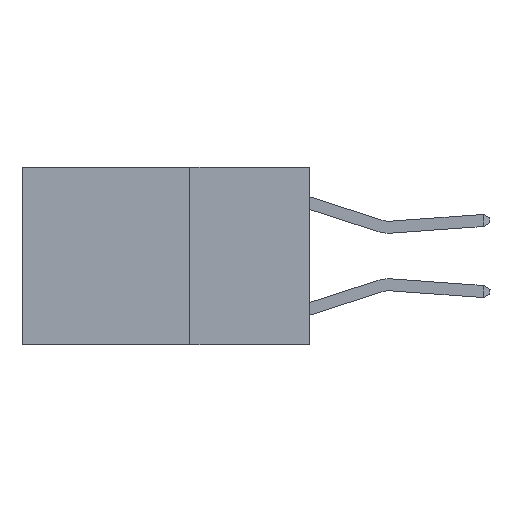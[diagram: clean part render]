
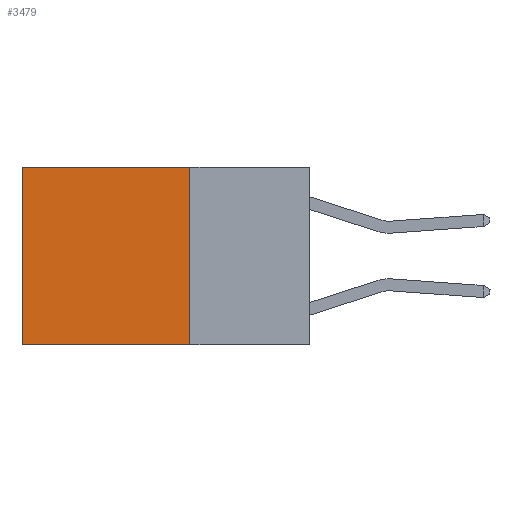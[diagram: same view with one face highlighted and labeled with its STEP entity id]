
A CAD part, left-side view. The second image highlights one B-rep face of the part: STEP entity #3479.
In plain terms, the highlighted planar face has unit normal (-1, 0, 0).
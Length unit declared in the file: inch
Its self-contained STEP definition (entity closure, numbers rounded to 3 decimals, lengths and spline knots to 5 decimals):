
#15 = AXIS2_PLACEMENT_3D ( 'NONE', #1675, #5451, #829 ) ;
#39 = PLANE ( 'NONE',  #15 ) ;
#236 = EDGE_CURVE ( 'NONE', #6786, #7391, #913, .T. ) ;
#303 = VERTEX_POINT ( 'NONE', #6705 ) ;
#782 = EDGE_CURVE ( 'NONE', #6786, #303, #9346, .T. ) ;
#812 = ORIENTED_EDGE ( 'NONE', *, *, #9551, .T. ) ;
#829 = DIRECTION ( 'NONE',  ( 0., 0., -1. ) ) ;
#878 = ORIENTED_EDGE ( 'NONE', *, *, #782, .F. ) ;
#913 = LINE ( 'NONE', #9697, #4128 ) ;
#1272 = CARTESIAN_POINT ( 'NONE',  ( 0.2625, 0.25, -0.37 ) ) ;
#1431 = EDGE_CURVE ( 'NONE', #303, #6467, #4686, .T. ) ;
#1623 = ORIENTED_EDGE ( 'NONE', *, *, #236, .T. ) ;
#1675 = CARTESIAN_POINT ( 'NONE',  ( 0.2625, 0.25, 0. ) ) ;
#2903 = VECTOR ( 'NONE', #3567, 39.37008 ) ;
#3479 = ADVANCED_FACE ( 'NONE', ( #6598 ), #39, .F. ) ;
#3567 = DIRECTION ( 'NONE',  ( 0., 1., 0. ) ) ;
#3615 = CARTESIAN_POINT ( 'NONE',  ( 0.2625, 0.6, -0.37 ) ) ;
#3731 = VECTOR ( 'NONE', #3846, 39.37008 ) ;
#3844 = LINE ( 'NONE', #5351, #3731 ) ;
#3846 = DIRECTION ( 'NONE',  ( 0., 0., -1. ) ) ;
#4128 = VECTOR ( 'NONE', #5115, 39.37008 ) ;
#4686 = LINE ( 'NONE', #1272, #2903 ) ;
#5115 = DIRECTION ( 'NONE',  ( 0., 1., 0. ) ) ;
#5351 = CARTESIAN_POINT ( 'NONE',  ( 0.2625, 0.6, 0. ) ) ;
#5451 = DIRECTION ( 'NONE',  ( 1., 0., 0. ) ) ;
#6374 = CARTESIAN_POINT ( 'NONE',  ( 0.2625, 0.6, 0. ) ) ;
#6388 = VECTOR ( 'NONE', #8823, 39.37008 ) ;
#6467 = VERTEX_POINT ( 'NONE', #3615 ) ;
#6598 = FACE_OUTER_BOUND ( 'NONE', #7121, .T. ) ;
#6705 = CARTESIAN_POINT ( 'NONE',  ( 0.2625, 0.25, -0.37 ) ) ;
#6786 = VERTEX_POINT ( 'NONE', #7008 ) ;
#7008 = CARTESIAN_POINT ( 'NONE',  ( 0.2625, 0.25, 0. ) ) ;
#7121 = EDGE_LOOP ( 'NONE', ( #812, #8252, #878, #1623 ) ) ;
#7217 = CARTESIAN_POINT ( 'NONE',  ( 0.2625, 0.25, 0. ) ) ;
#7391 = VERTEX_POINT ( 'NONE', #6374 ) ;
#8252 = ORIENTED_EDGE ( 'NONE', *, *, #1431, .F. ) ;
#8823 = DIRECTION ( 'NONE',  ( 0., 0., -1. ) ) ;
#9346 = LINE ( 'NONE', #7217, #6388 ) ;
#9551 = EDGE_CURVE ( 'NONE', #7391, #6467, #3844, .T. ) ;
#9697 = CARTESIAN_POINT ( 'NONE',  ( 0.2625, 0.25, 0. ) ) ;
